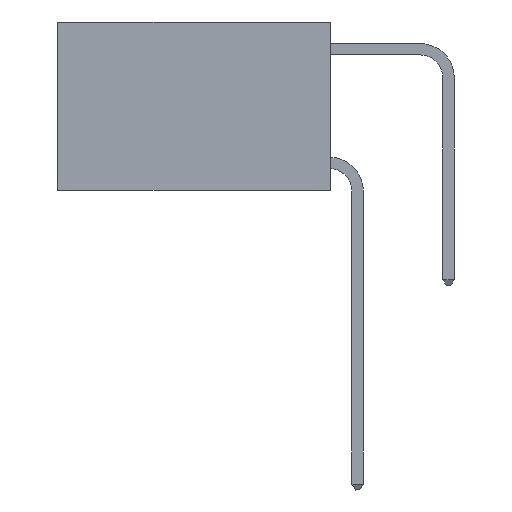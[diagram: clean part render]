
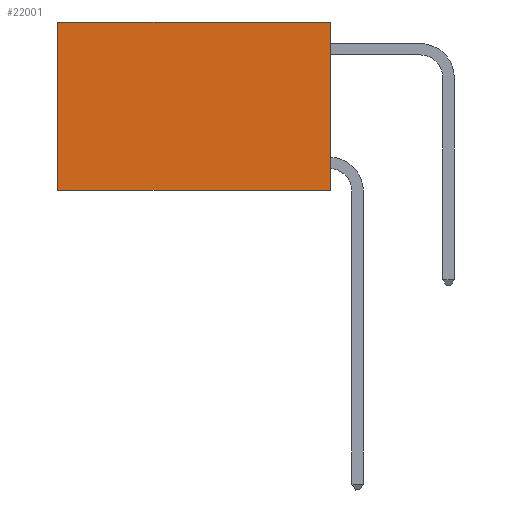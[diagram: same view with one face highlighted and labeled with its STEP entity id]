
A CAD part, left-side view. The second image highlights one B-rep face of the part: STEP entity #22001.
In plain terms, the highlighted planar face has unit normal (-1, 0, 0).
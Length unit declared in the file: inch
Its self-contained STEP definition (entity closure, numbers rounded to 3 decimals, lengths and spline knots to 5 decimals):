
#1598 = ORIENTED_EDGE ( 'NONE', *, *, #11095, .F. ) ;
#1868 = ORIENTED_EDGE ( 'NONE', *, *, #23489, .T. ) ;
#2437 = ORIENTED_EDGE ( 'NONE', *, *, #5658, .F. ) ;
#3828 = CARTESIAN_POINT ( 'NONE',  ( 0.2625, 0., -0.37 ) ) ;
#4128 = VERTEX_POINT ( 'NONE', #23308 ) ;
#4524 = VECTOR ( 'NONE', #17040, 39.37008 ) ;
#5658 = EDGE_CURVE ( 'NONE', #13942, #15926, #20241, .T. ) ;
#6305 = DIRECTION ( 'NONE',  ( 1., 0., 0. ) ) ;
#6546 = ORIENTED_EDGE ( 'NONE', *, *, #9702, .T. ) ;
#7059 = DIRECTION ( 'NONE',  ( 0., 0., -1. ) ) ;
#9052 = CARTESIAN_POINT ( 'NONE',  ( 0.2625, 0., -0.37 ) ) ;
#9532 = LINE ( 'NONE', #24200, #26005 ) ;
#9702 = EDGE_CURVE ( 'NONE', #4128, #15926, #26730, .T. ) ;
#11095 = EDGE_CURVE ( 'NONE', #27518, #13942, #9532, .T. ) ;
#11169 = FACE_OUTER_BOUND ( 'NONE', #17677, .T. ) ;
#13942 = VERTEX_POINT ( 'NONE', #3828 ) ;
#14201 = CARTESIAN_POINT ( 'NONE',  ( 0.2625, 0., 0. ) ) ;
#14875 = CARTESIAN_POINT ( 'NONE',  ( 0.2625, 0.6, 0. ) ) ;
#15504 = CARTESIAN_POINT ( 'NONE',  ( 0.2625, 0., 0. ) ) ;
#15926 = VERTEX_POINT ( 'NONE', #25141 ) ;
#17040 = DIRECTION ( 'NONE',  ( 0., 0., -1. ) ) ;
#17677 = EDGE_LOOP ( 'NONE', ( #6546, #2437, #1598, #1868 ) ) ;
#17784 = DIRECTION ( 'NONE',  ( 0., 1., 0. ) ) ;
#18684 = PLANE ( 'NONE',  #23441 ) ;
#19244 = CARTESIAN_POINT ( 'NONE',  ( 0.2625, 0., 0. ) ) ;
#19794 = DIRECTION ( 'NONE',  ( 0., 1., 0. ) ) ;
#20241 = LINE ( 'NONE', #9052, #25280 ) ;
#21375 = DIRECTION ( 'NONE',  ( 0., 0., -1. ) ) ;
#22001 = ADVANCED_FACE ( 'NONE', ( #11169 ), #18684, .F. ) ;
#23308 = CARTESIAN_POINT ( 'NONE',  ( 0.2625, 0.6, 0. ) ) ;
#23441 = AXIS2_PLACEMENT_3D ( 'NONE', #19244, #6305, #21375 ) ;
#23489 = EDGE_CURVE ( 'NONE', #27518, #4128, #25915, .T. ) ;
#24200 = CARTESIAN_POINT ( 'NONE',  ( 0.2625, 0., 0. ) ) ;
#25141 = CARTESIAN_POINT ( 'NONE',  ( 0.2625, 0.6, -0.37 ) ) ;
#25252 = VECTOR ( 'NONE', #17784, 39.37008 ) ;
#25280 = VECTOR ( 'NONE', #19794, 39.37008 ) ;
#25915 = LINE ( 'NONE', #15504, #25252 ) ;
#26005 = VECTOR ( 'NONE', #7059, 39.37008 ) ;
#26730 = LINE ( 'NONE', #14875, #4524 ) ;
#27518 = VERTEX_POINT ( 'NONE', #14201 ) ;
